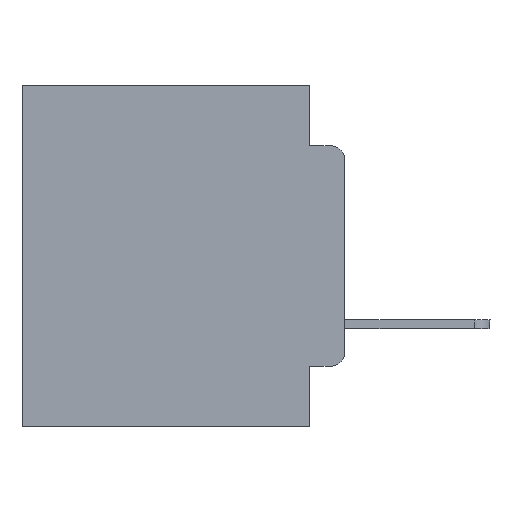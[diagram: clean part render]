
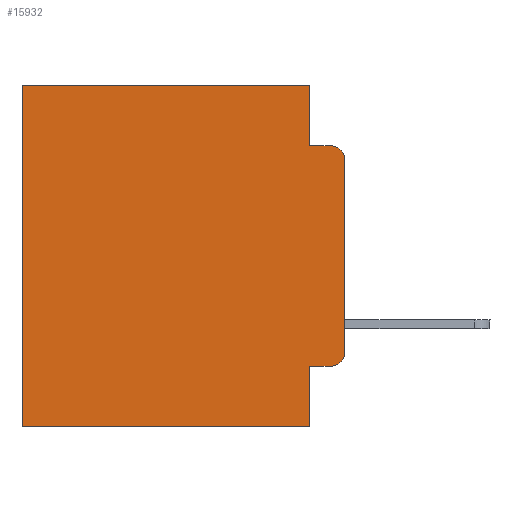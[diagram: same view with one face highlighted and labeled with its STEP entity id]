
A CAD part, left-side view. The second image highlights one B-rep face of the part: STEP entity #15932.
In plain terms, the highlighted planar face has unit normal (-1, 0, 0).
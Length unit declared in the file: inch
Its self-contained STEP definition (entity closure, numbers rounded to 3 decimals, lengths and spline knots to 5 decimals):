
#168 = FACE_OUTER_BOUND ( 'NONE', #22615, .T. ) ;
#862 = DIRECTION ( 'NONE',  ( -1., 0., 0. ) ) ;
#1328 = CARTESIAN_POINT ( 'NONE',  ( 0.298, 0.051, -0.5 ) ) ;
#1448 = VERTEX_POINT ( 'NONE', #23953 ) ;
#1672 = DIRECTION ( 'NONE',  ( 0., 0., -1. ) ) ;
#1736 = CARTESIAN_POINT ( 'NONE',  ( 0.298, 0.473, -0.5 ) ) ;
#2989 = CIRCLE ( 'NONE', #18605, 0.02 ) ;
#3333 = ORIENTED_EDGE ( 'NONE', *, *, #11986, .T. ) ;
#3828 = EDGE_CURVE ( 'NONE', #21836, #11603, #14785, .T. ) ;
#3871 = DIRECTION ( 'NONE',  ( 0., 0., -1. ) ) ;
#3985 = CARTESIAN_POINT ( 'NONE',  ( 0.298, 0., 0. ) ) ;
#4468 = VECTOR ( 'NONE', #9592, 39.37008 ) ;
#4524 = VERTEX_POINT ( 'NONE', #8456 ) ;
#4727 = DIRECTION ( 'NONE',  ( 0., -1., 0. ) ) ;
#5234 = CARTESIAN_POINT ( 'NONE',  ( 0.298, 0., -0.5 ) ) ;
#5235 = CARTESIAN_POINT ( 'NONE',  ( 0.298, 0.02, -0.3915 ) ) ;
#5288 = VECTOR ( 'NONE', #6761, 39.37008 ) ;
#5755 = VECTOR ( 'NONE', #13548, 39.37008 ) ;
#6173 = DIRECTION ( 'NONE',  ( 1., 0., 0. ) ) ;
#6761 = DIRECTION ( 'NONE',  ( 0., 0., -1. ) ) ;
#7433 = ORIENTED_EDGE ( 'NONE', *, *, #19774, .F. ) ;
#7822 = DIRECTION ( 'NONE',  ( 0., 0., -1. ) ) ;
#8456 = CARTESIAN_POINT ( 'NONE',  ( 0.298, 0., -0.3915 ) ) ;
#8487 = PLANE ( 'NONE',  #10049 ) ;
#8554 = VERTEX_POINT ( 'NONE', #1328 ) ;
#9592 = DIRECTION ( 'NONE',  ( 0., 1., 0. ) ) ;
#9620 = CARTESIAN_POINT ( 'NONE',  ( 0.298, 0.051, -0.0885 ) ) ;
#9644 = VECTOR ( 'NONE', #1672, 39.37008 ) ;
#10049 = AXIS2_PLACEMENT_3D ( 'NONE', #3985, #6173, #12282 ) ;
#10351 = VECTOR ( 'NONE', #3871, 39.37008 ) ;
#10923 = VERTEX_POINT ( 'NONE', #1736 ) ;
#11280 = VECTOR ( 'NONE', #4727, 39.37008 ) ;
#11282 = LINE ( 'NONE', #15493, #25565 ) ;
#11589 = EDGE_CURVE ( 'NONE', #11603, #4524, #24232, .T. ) ;
#11603 = VERTEX_POINT ( 'NONE', #23548 ) ;
#11986 = EDGE_CURVE ( 'NONE', #26673, #12997, #11282, .T. ) ;
#12040 = LINE ( 'NONE', #9620, #5755 ) ;
#12241 = EDGE_CURVE ( 'NONE', #15796, #1448, #2989, .T. ) ;
#12282 = DIRECTION ( 'NONE',  ( 0., 0., -1. ) ) ;
#12522 = ORIENTED_EDGE ( 'NONE', *, *, #11589, .T. ) ;
#12997 = VERTEX_POINT ( 'NONE', #21068 ) ;
#13043 = ORIENTED_EDGE ( 'NONE', *, *, #24546, .F. ) ;
#13272 = CARTESIAN_POINT ( 'NONE',  ( 0.298, 0.473, 0. ) ) ;
#13548 = DIRECTION ( 'NONE',  ( 0., -1., 0. ) ) ;
#14030 = ORIENTED_EDGE ( 'NONE', *, *, #15776, .F. ) ;
#14645 = DIRECTION ( 'NONE',  ( -1., 0., 0. ) ) ;
#14785 = LINE ( 'NONE', #23051, #11280 ) ;
#15296 = EDGE_CURVE ( 'NONE', #25205, #1448, #12040, .T. ) ;
#15493 = CARTESIAN_POINT ( 'NONE',  ( 0.298, 0., 0. ) ) ;
#15776 = EDGE_CURVE ( 'NONE', #8554, #10923, #20119, .T. ) ;
#15796 = VERTEX_POINT ( 'NONE', #24228 ) ;
#15932 = ADVANCED_FACE ( 'NONE', ( #168 ), #8487, .F. ) ;
#15964 = EDGE_CURVE ( 'NONE', #21836, #8554, #18637, .T. ) ;
#16220 = CARTESIAN_POINT ( 'NONE',  ( 0.298, 0., 0. ) ) ;
#16446 = EDGE_CURVE ( 'NONE', #12997, #10923, #19359, .T. ) ;
#16489 = LINE ( 'NONE', #16220, #10351 ) ;
#17573 = DIRECTION ( 'NONE',  ( 0., 0., -1. ) ) ;
#17993 = VECTOR ( 'NONE', #7822, 39.37008 ) ;
#18605 = AXIS2_PLACEMENT_3D ( 'NONE', #25638, #14645, #21284 ) ;
#18637 = LINE ( 'NONE', #25034, #9644 ) ;
#19359 = LINE ( 'NONE', #13272, #5288 ) ;
#19774 = EDGE_CURVE ( 'NONE', #26673, #25205, #22052, .T. ) ;
#20064 = ORIENTED_EDGE ( 'NONE', *, *, #16446, .T. ) ;
#20119 = LINE ( 'NONE', #5234, #4468 ) ;
#21068 = CARTESIAN_POINT ( 'NONE',  ( 0.298, 0.473, 0. ) ) ;
#21086 = CARTESIAN_POINT ( 'NONE',  ( 0.298, 0.051, -0.0885 ) ) ;
#21284 = DIRECTION ( 'NONE',  ( 0., 0., -1. ) ) ;
#21394 = CARTESIAN_POINT ( 'NONE',  ( 0.298, 0.051, 0. ) ) ;
#21799 = ORIENTED_EDGE ( 'NONE', *, *, #12241, .T. ) ;
#21836 = VERTEX_POINT ( 'NONE', #22618 ) ;
#21837 = ORIENTED_EDGE ( 'NONE', *, *, #15964, .F. ) ;
#22052 = LINE ( 'NONE', #24637, #17993 ) ;
#22615 = EDGE_LOOP ( 'NONE', ( #13043, #21799, #24110, #7433, #3333, #20064, #14030, #21837, #24385, #12522 ) ) ;
#22618 = CARTESIAN_POINT ( 'NONE',  ( 0.298, 0.051, -0.4115 ) ) ;
#23051 = CARTESIAN_POINT ( 'NONE',  ( 0.298, 0.051, -0.4115 ) ) ;
#23548 = CARTESIAN_POINT ( 'NONE',  ( 0.298, 0.02, -0.4115 ) ) ;
#23897 = DIRECTION ( 'NONE',  ( 0., 1., 0. ) ) ;
#23953 = CARTESIAN_POINT ( 'NONE',  ( 0.298, 0.02, -0.0885 ) ) ;
#24110 = ORIENTED_EDGE ( 'NONE', *, *, #15296, .F. ) ;
#24228 = CARTESIAN_POINT ( 'NONE',  ( 0.298, 0., -0.1085 ) ) ;
#24232 = CIRCLE ( 'NONE', #25096, 0.02 ) ;
#24385 = ORIENTED_EDGE ( 'NONE', *, *, #3828, .T. ) ;
#24546 = EDGE_CURVE ( 'NONE', #15796, #4524, #16489, .T. ) ;
#24637 = CARTESIAN_POINT ( 'NONE',  ( 0.298, 0.051, 0. ) ) ;
#25034 = CARTESIAN_POINT ( 'NONE',  ( 0.298, 0.051, 0. ) ) ;
#25096 = AXIS2_PLACEMENT_3D ( 'NONE', #5235, #862, #17573 ) ;
#25205 = VERTEX_POINT ( 'NONE', #21086 ) ;
#25565 = VECTOR ( 'NONE', #23897, 39.37008 ) ;
#25638 = CARTESIAN_POINT ( 'NONE',  ( 0.298, 0.02, -0.1085 ) ) ;
#26673 = VERTEX_POINT ( 'NONE', #21394 ) ;
